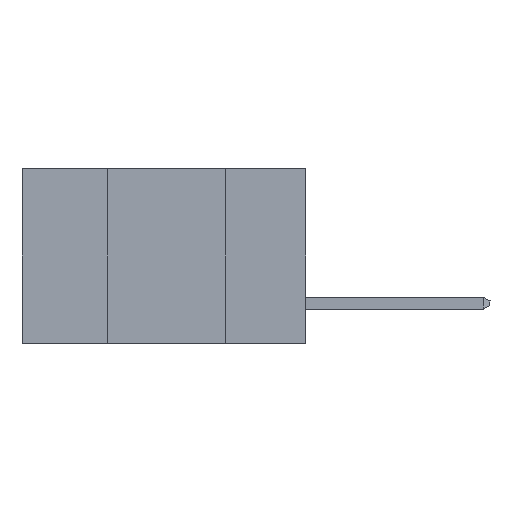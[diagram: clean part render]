
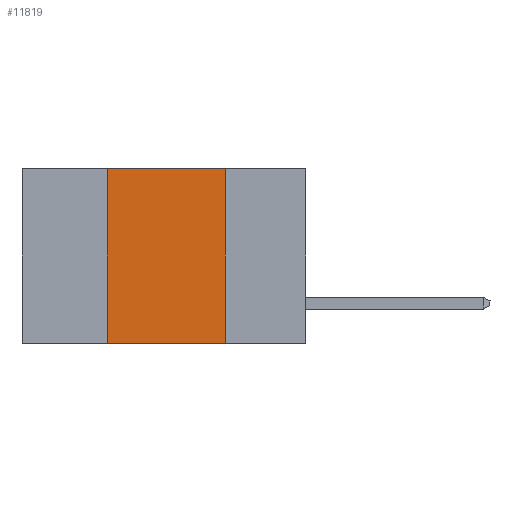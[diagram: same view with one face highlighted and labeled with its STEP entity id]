
A CAD part, left-side view. The second image highlights one B-rep face of the part: STEP entity #11819.
In plain terms, the highlighted planar face has unit normal (-1, 0, 0).
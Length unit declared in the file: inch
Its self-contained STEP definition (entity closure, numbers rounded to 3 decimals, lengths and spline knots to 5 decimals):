
#473 = LINE ( 'NONE', #9462, #18664 ) ;
#843 = CARTESIAN_POINT ( 'NONE',  ( 0., 0.42, -0.37 ) ) ;
#2160 = CARTESIAN_POINT ( 'NONE',  ( 0., 0.42, 0. ) ) ;
#3689 = DIRECTION ( 'NONE',  ( 0., -1., 0. ) ) ;
#4061 = VECTOR ( 'NONE', #4477, 39.37008 ) ;
#4477 = DIRECTION ( 'NONE',  ( 0., 0., -1. ) ) ;
#5164 = VECTOR ( 'NONE', #21705, 39.37008 ) ;
#5205 = PLANE ( 'NONE',  #17029 ) ;
#6031 = DIRECTION ( 'NONE',  ( 0., -1., 0. ) ) ;
#6709 = VERTEX_POINT ( 'NONE', #20006 ) ;
#6764 = CARTESIAN_POINT ( 'NONE',  ( 0., 0.6, -0.37 ) ) ;
#7098 = ORIENTED_EDGE ( 'NONE', *, *, #21187, .F. ) ;
#7814 = ORIENTED_EDGE ( 'NONE', *, *, #13573, .F. ) ;
#9291 = EDGE_CURVE ( 'NONE', #17469, #16687, #19656, .T. ) ;
#9364 = VERTEX_POINT ( 'NONE', #2160 ) ;
#9462 = CARTESIAN_POINT ( 'NONE',  ( 0., 0.6, 0. ) ) ;
#9774 = CARTESIAN_POINT ( 'NONE',  ( 0., 0.17, 0. ) ) ;
#10605 = CARTESIAN_POINT ( 'NONE',  ( 0., 0.17, -0.37 ) ) ;
#11013 = ORIENTED_EDGE ( 'NONE', *, *, #20383, .F. ) ;
#11819 = ADVANCED_FACE ( 'NONE', ( #12727 ), #5205, .F. ) ;
#12523 = ORIENTED_EDGE ( 'NONE', *, *, #9291, .T. ) ;
#12727 = FACE_OUTER_BOUND ( 'NONE', #13047, .T. ) ;
#13047 = EDGE_LOOP ( 'NONE', ( #11013, #7098, #7814, #12523 ) ) ;
#13573 = EDGE_CURVE ( 'NONE', #17469, #9364, #19249, .T. ) ;
#14301 = LINE ( 'NONE', #9774, #4061 ) ;
#15821 = VECTOR ( 'NONE', #3689, 39.37008 ) ;
#15871 = DIRECTION ( 'NONE',  ( 0., 0., -1. ) ) ;
#16687 = VERTEX_POINT ( 'NONE', #10605 ) ;
#17029 = AXIS2_PLACEMENT_3D ( 'NONE', #19260, #21163, #15871 ) ;
#17469 = VERTEX_POINT ( 'NONE', #843 ) ;
#18194 = CARTESIAN_POINT ( 'NONE',  ( 0., 0.42, 0. ) ) ;
#18664 = VECTOR ( 'NONE', #6031, 39.37008 ) ;
#19249 = LINE ( 'NONE', #18194, #5164 ) ;
#19260 = CARTESIAN_POINT ( 'NONE',  ( 0., 0.6, 0. ) ) ;
#19656 = LINE ( 'NONE', #6764, #15821 ) ;
#20006 = CARTESIAN_POINT ( 'NONE',  ( 0., 0.17, 0. ) ) ;
#20383 = EDGE_CURVE ( 'NONE', #6709, #16687, #14301, .T. ) ;
#21163 = DIRECTION ( 'NONE',  ( 1., 0., 0. ) ) ;
#21187 = EDGE_CURVE ( 'NONE', #9364, #6709, #473, .T. ) ;
#21705 = DIRECTION ( 'NONE',  ( 0., 0., 1. ) ) ;
